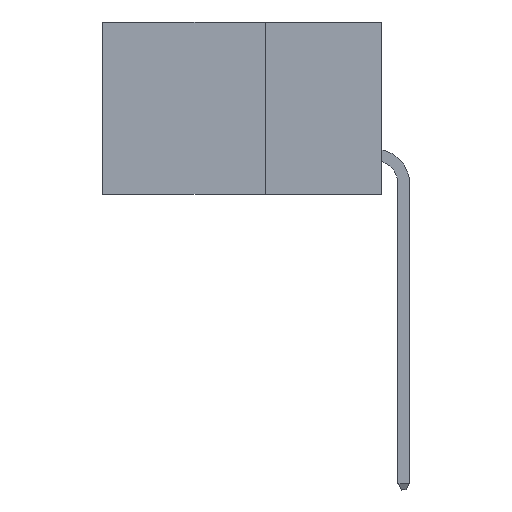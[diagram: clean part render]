
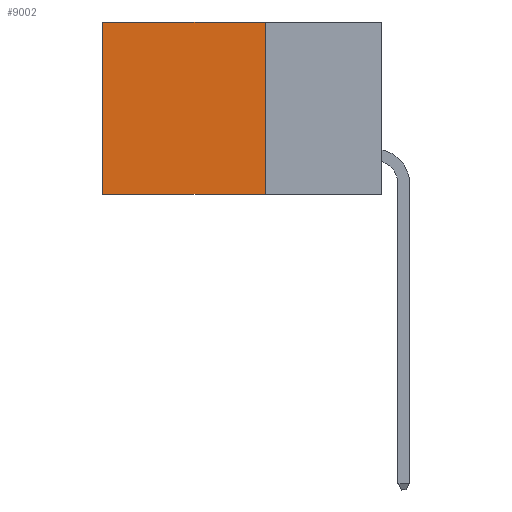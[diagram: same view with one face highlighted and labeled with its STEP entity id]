
A CAD part, left-side view. The second image highlights one B-rep face of the part: STEP entity #9002.
In plain terms, the highlighted planar face has unit normal (-1, 0, 0).
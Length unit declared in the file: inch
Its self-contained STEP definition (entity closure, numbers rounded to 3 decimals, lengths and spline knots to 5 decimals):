
#753 = EDGE_CURVE ( 'NONE', #17747, #9451, #7824, .T. ) ;
#3195 = CARTESIAN_POINT ( 'NONE',  ( 0.2875, 0.25, 0. ) ) ;
#3203 = DIRECTION ( 'NONE',  ( 1., 0., 0. ) ) ;
#5262 = ORIENTED_EDGE ( 'NONE', *, *, #18742, .F. ) ;
#5841 = VECTOR ( 'NONE', #18879, 39.37008 ) ;
#6654 = CARTESIAN_POINT ( 'NONE',  ( 0.2875, 0.25, -0.37 ) ) ;
#6882 = ORIENTED_EDGE ( 'NONE', *, *, #753, .F. ) ;
#7102 = EDGE_CURVE ( 'NONE', #15846, #9970, #10061, .T. ) ;
#7138 = CARTESIAN_POINT ( 'NONE',  ( 0.2875, 0.25, 0. ) ) ;
#7412 = EDGE_LOOP ( 'NONE', ( #16284, #6882, #5262, #11923 ) ) ;
#7495 = CARTESIAN_POINT ( 'NONE',  ( 0.2875, 0.6, 0. ) ) ;
#7824 = LINE ( 'NONE', #13252, #8336 ) ;
#7918 = VECTOR ( 'NONE', #13420, 39.37008 ) ;
#8011 = DIRECTION ( 'NONE',  ( 0., 0., -1. ) ) ;
#8336 = VECTOR ( 'NONE', #17707, 39.37008 ) ;
#9002 = ADVANCED_FACE ( 'NONE', ( #9456 ), #17272, .F. ) ;
#9451 = VERTEX_POINT ( 'NONE', #16182 ) ;
#9456 = FACE_OUTER_BOUND ( 'NONE', #7412, .T. ) ;
#9970 = VERTEX_POINT ( 'NONE', #7495 ) ;
#10032 = VECTOR ( 'NONE', #15648, 39.37008 ) ;
#10061 = LINE ( 'NONE', #3195, #5841 ) ;
#11923 = ORIENTED_EDGE ( 'NONE', *, *, #7102, .T. ) ;
#12087 = EDGE_CURVE ( 'NONE', #9970, #9451, #14001, .T. ) ;
#13252 = CARTESIAN_POINT ( 'NONE',  ( 0.2875, 0.25, -0.37 ) ) ;
#13420 = DIRECTION ( 'NONE',  ( 0., 0., -1. ) ) ;
#13827 = LINE ( 'NONE', #14900, #7918 ) ;
#13892 = CARTESIAN_POINT ( 'NONE',  ( 0.2875, 0.6, 0. ) ) ;
#14001 = LINE ( 'NONE', #13892, #10032 ) ;
#14900 = CARTESIAN_POINT ( 'NONE',  ( 0.2875, 0.25, 0. ) ) ;
#15648 = DIRECTION ( 'NONE',  ( 0., 0., -1. ) ) ;
#15846 = VERTEX_POINT ( 'NONE', #7138 ) ;
#16182 = CARTESIAN_POINT ( 'NONE',  ( 0.2875, 0.6, -0.37 ) ) ;
#16284 = ORIENTED_EDGE ( 'NONE', *, *, #12087, .T. ) ;
#17272 = PLANE ( 'NONE',  #17711 ) ;
#17484 = CARTESIAN_POINT ( 'NONE',  ( 0.2875, 0.25, 0. ) ) ;
#17707 = DIRECTION ( 'NONE',  ( 0., 1., 0. ) ) ;
#17711 = AXIS2_PLACEMENT_3D ( 'NONE', #17484, #3203, #8011 ) ;
#17747 = VERTEX_POINT ( 'NONE', #6654 ) ;
#18742 = EDGE_CURVE ( 'NONE', #15846, #17747, #13827, .T. ) ;
#18879 = DIRECTION ( 'NONE',  ( 0., 1., 0. ) ) ;
